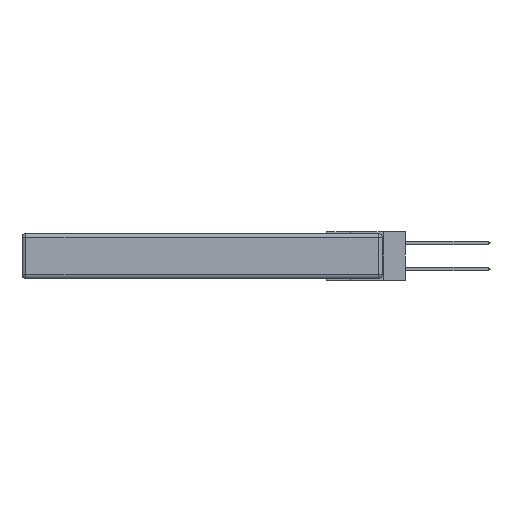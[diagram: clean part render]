
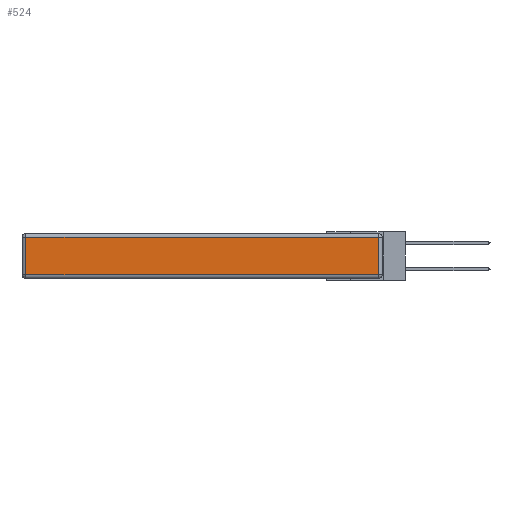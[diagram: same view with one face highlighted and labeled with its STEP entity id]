
A CAD part, left-side view. The second image highlights one B-rep face of the part: STEP entity #524.
In plain terms, the highlighted planar face has unit normal (-1, 0, 0).
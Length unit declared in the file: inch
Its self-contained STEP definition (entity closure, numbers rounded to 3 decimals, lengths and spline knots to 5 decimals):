
#74 = VECTOR ( 'NONE', #14297, 39.37008 ) ;
#524 = ADVANCED_FACE ( 'NONE', ( #1098 ), #4035, .T. ) ;
#1098 = FACE_OUTER_BOUND ( 'NONE', #1904, .T. ) ;
#1542 = VERTEX_POINT ( 'NONE', #20187 ) ;
#1904 = EDGE_LOOP ( 'NONE', ( #29982, #17201, #3792, #25306 ) ) ;
#2962 = VERTEX_POINT ( 'NONE', #16936 ) ;
#3646 = EDGE_CURVE ( 'NONE', #27328, #1542, #10673, .T. ) ;
#3792 = ORIENTED_EDGE ( 'NONE', *, *, #7072, .T. ) ;
#3919 = LINE ( 'NONE', #30274, #11244 ) ;
#4035 = PLANE ( 'NONE',  #13717 ) ;
#7072 = EDGE_CURVE ( 'NONE', #19365, #27328, #30140, .T. ) ;
#9186 = CARTESIAN_POINT ( 'NONE',  ( 0., 0., -0.343 ) ) ;
#10673 = LINE ( 'NONE', #27405, #74 ) ;
#11244 = VECTOR ( 'NONE', #22358, 39.37008 ) ;
#12944 = CARTESIAN_POINT ( 'NONE',  ( 0., 0.03, -0.03 ) ) ;
#13717 = AXIS2_PLACEMENT_3D ( 'NONE', #9186, #24696, #32382 ) ;
#14297 = DIRECTION ( 'NONE',  ( 0., 0., -1. ) ) ;
#14497 = VECTOR ( 'NONE', #29157, 39.37008 ) ;
#14746 = DIRECTION ( 'NONE',  ( 0., 1., 0. ) ) ;
#16936 = CARTESIAN_POINT ( 'NONE',  ( 0., 0.03, -0.313 ) ) ;
#17201 = ORIENTED_EDGE ( 'NONE', *, *, #28384, .T. ) ;
#19365 = VERTEX_POINT ( 'NONE', #12944 ) ;
#20187 = CARTESIAN_POINT ( 'NONE',  ( 0., 2.72, -0.313 ) ) ;
#22358 = DIRECTION ( 'NONE',  ( 0., -1., 0. ) ) ;
#22724 = CARTESIAN_POINT ( 'NONE',  ( 0., 2.72, -0.03 ) ) ;
#24696 = DIRECTION ( 'NONE',  ( -1., 0., 0. ) ) ;
#24926 = CARTESIAN_POINT ( 'NONE',  ( 0., 2.75, -0.03 ) ) ;
#25306 = ORIENTED_EDGE ( 'NONE', *, *, #3646, .T. ) ;
#25835 = LINE ( 'NONE', #32134, #14497 ) ;
#27328 = VERTEX_POINT ( 'NONE', #22724 ) ;
#27405 = CARTESIAN_POINT ( 'NONE',  ( 0., 2.72, -0.343 ) ) ;
#28384 = EDGE_CURVE ( 'NONE', #2962, #19365, #25835, .T. ) ;
#28580 = EDGE_CURVE ( 'NONE', #1542, #2962, #3919, .T. ) ;
#29157 = DIRECTION ( 'NONE',  ( 0., 0., 1. ) ) ;
#29332 = VECTOR ( 'NONE', #14746, 39.37008 ) ;
#29982 = ORIENTED_EDGE ( 'NONE', *, *, #28580, .T. ) ;
#30140 = LINE ( 'NONE', #24926, #29332 ) ;
#30274 = CARTESIAN_POINT ( 'NONE',  ( 0., 0., -0.313 ) ) ;
#32134 = CARTESIAN_POINT ( 'NONE',  ( 0., 0.03, -0.343 ) ) ;
#32382 = DIRECTION ( 'NONE',  ( 0., 0., 1. ) ) ;
